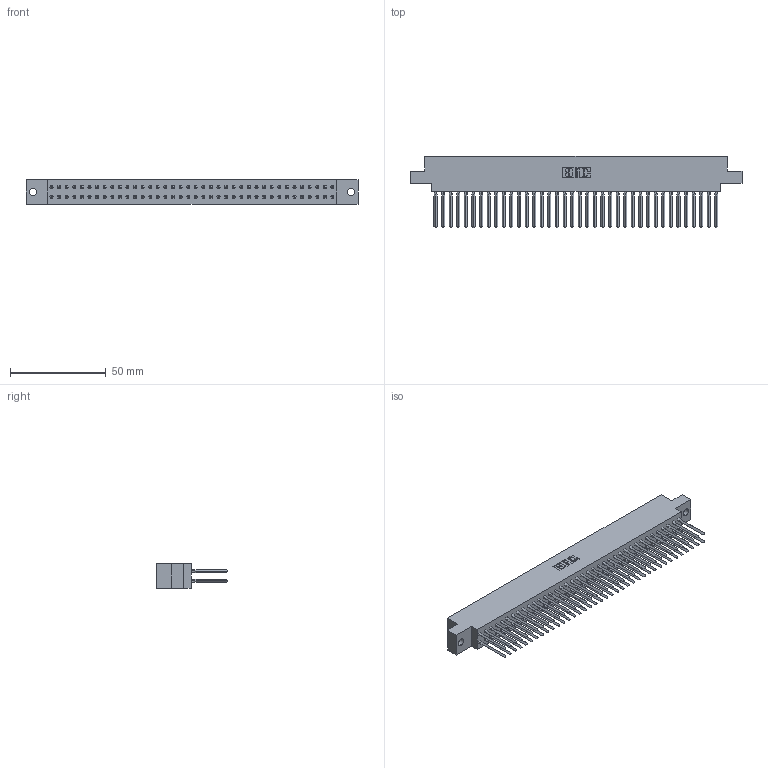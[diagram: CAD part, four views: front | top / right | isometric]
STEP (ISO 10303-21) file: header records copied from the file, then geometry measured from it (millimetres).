
FILE_DESCRIPTION (( 'STEP AP203' ), '1' );
FILE_NAME ('317-076-542-804.STEP', '2020-02-28T08:24:20', ( '' ), ( '' ), 'SwSTEP 2.0', 'SolidWorks 2016', '' );
FILE_SCHEMA (( 'CONFIG_CONTROL_DESIGN' ));
Length unit declared in the file: inch
Products named in the file (3): 317-290-003_542; 317-076-542-804; 317 Part_.156 Dia - TH
Assembly tree (77 placements, depth 2):
  317-076-542-804
    317 Part_.156 Dia - TH
    317-290-003_542  x76
Bounding box: 173.28 x 37.34 x 12.7 mm (x, y, z)
Volume: 28159.6 mm3; surface area: 38847.2 mm2
Topology: 77 solids, 77 shells, 4434 faces, 12435 edges, 7934 vertices
Faces by surface type: plane 3554, cylinder 576, bspline 304
Entity records: 54507 total; most frequent: CARTESIAN_POINT 9757, ORIENTED_EDGE 9420, DIRECTION 7930, EDGE_CURVE 4710, VECTOR 4540, LINE 4540, VERTEX_POINT 3134, AXIS2_PLACEMENT_3D 1695
